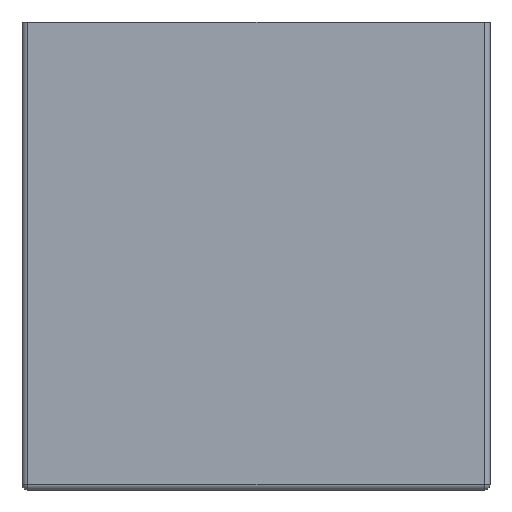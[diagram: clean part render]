
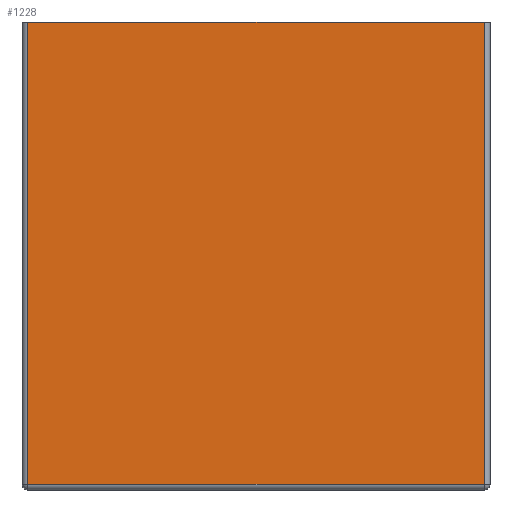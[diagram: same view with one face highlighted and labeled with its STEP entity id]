
A CAD part, front view. The second image highlights one B-rep face of the part: STEP entity #1228.
In plain terms, the highlighted planar face has unit normal (0, -1, 0).
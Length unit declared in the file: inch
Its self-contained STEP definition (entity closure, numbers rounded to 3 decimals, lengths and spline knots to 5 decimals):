
#47=PLANE('',#1372);
#158=LINE('',#2035,#276);
#164=LINE('',#2062,#282);
#173=LINE('',#2099,#291);
#186=LINE('',#2130,#304);
#276=VECTOR('',#1613,0.3937);
#282=VECTOR('',#1647,0.3937);
#291=VECTOR('',#1692,0.3937);
#304=VECTOR('',#1729,0.3937);
#384=FACE_OUTER_BOUND('',#463,.T.);
#463=EDGE_LOOP('',(#1119,#1120,#1121,#1122));
#584=VERTEX_POINT('',#2025);
#586=VERTEX_POINT('',#2031);
#593=VERTEX_POINT('',#2056);
#604=VERTEX_POINT('',#2097);
#732=EDGE_CURVE('',#584,#586,#158,.T.);
#746=EDGE_CURVE('',#593,#584,#164,.T.);
#764=EDGE_CURVE('',#604,#593,#173,.T.);
#780=EDGE_CURVE('',#604,#586,#186,.T.);
#1119=ORIENTED_EDGE('',*,*,#764,.F.);
#1120=ORIENTED_EDGE('',*,*,#780,.T.);
#1121=ORIENTED_EDGE('',*,*,#732,.F.);
#1122=ORIENTED_EDGE('',*,*,#746,.F.);
#1228=ADVANCED_FACE('',(#384),#47,.F.);
#1372=AXIS2_PLACEMENT_3D('',#2136,#1738,#1739);
#1613=DIRECTION('',(0.,0.,1.));
#1647=DIRECTION('',(-1.,0.,0.));
#1692=DIRECTION('',(0.,0.,-1.));
#1729=DIRECTION('',(-1.,0.,0.));
#1738=DIRECTION('center_axis',(0.,1.,0.));
#1739=DIRECTION('ref_axis',(0.,0.,1.));
#2025=CARTESIAN_POINT('',(-1.975,0.,-1.975));
#2031=CARTESIAN_POINT('',(-1.975,0.,0.));
#2035=CARTESIAN_POINT('',(-1.975,0.,-1.5));
#2056=CARTESIAN_POINT('',(-0.025,0.,-1.975));
#2062=CARTESIAN_POINT('',(-0.5,0.,-1.975));
#2097=CARTESIAN_POINT('',(-0.025,0.,0.));
#2099=CARTESIAN_POINT('',(-0.025,0.,-0.5));
#2130=CARTESIAN_POINT('',(0.,0.,0.));
#2136=CARTESIAN_POINT('Origin',(-1.,0.,-1.));
